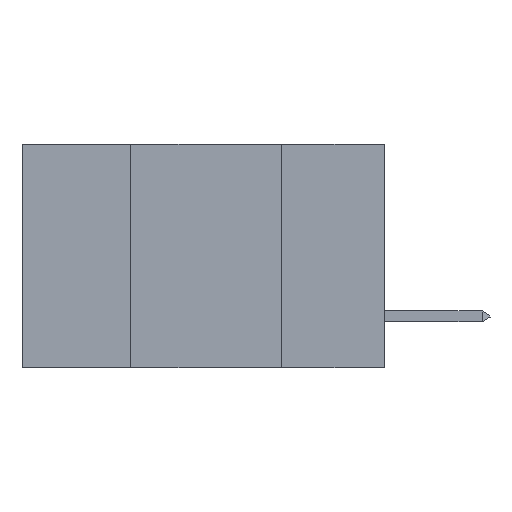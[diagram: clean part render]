
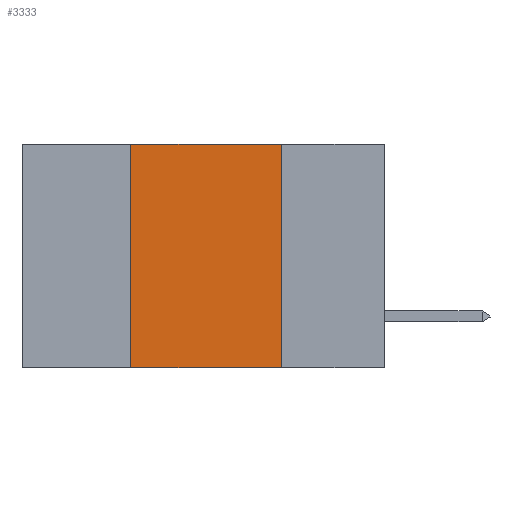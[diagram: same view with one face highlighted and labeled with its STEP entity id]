
A CAD part, left-side view. The second image highlights one B-rep face of the part: STEP entity #3333.
In plain terms, the highlighted planar face has unit normal (-1, 0, 0).
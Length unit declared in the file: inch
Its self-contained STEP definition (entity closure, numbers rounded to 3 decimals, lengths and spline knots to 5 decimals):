
#1678 = VERTEX_POINT ( 'NONE', #30557 ) ;
#2761 = DIRECTION ( 'NONE',  ( 0., -1., 0. ) ) ;
#3333 = ADVANCED_FACE ( 'NONE', ( #39121 ), #10931, .F. ) ;
#3868 = DIRECTION ( 'NONE',  ( 0., 0., -1. ) ) ;
#5580 = VECTOR ( 'NONE', #2761, 39.37008 ) ;
#7299 = CARTESIAN_POINT ( 'NONE',  ( 0., 0.17, 0. ) ) ;
#10762 = CARTESIAN_POINT ( 'NONE',  ( 0., 0.6, -0.37 ) ) ;
#10931 = PLANE ( 'NONE',  #16946 ) ;
#11097 = EDGE_CURVE ( 'NONE', #12855, #47499, #28608, .T. ) ;
#12492 = ORIENTED_EDGE ( 'NONE', *, *, #15811, .F. ) ;
#12855 = VERTEX_POINT ( 'NONE', #33168 ) ;
#14187 = DIRECTION ( 'NONE',  ( 0., -1., 0. ) ) ;
#14217 = CARTESIAN_POINT ( 'NONE',  ( 0., 0.42, 0. ) ) ;
#14856 = DIRECTION ( 'NONE',  ( 0., 0., -1. ) ) ;
#15482 = LINE ( 'NONE', #7299, #34998 ) ;
#15811 = EDGE_CURVE ( 'NONE', #47499, #33558, #34415, .T. ) ;
#16487 = DIRECTION ( 'NONE',  ( 0., 0., 1. ) ) ;
#16946 = AXIS2_PLACEMENT_3D ( 'NONE', #41458, #33560, #14856 ) ;
#19000 = EDGE_CURVE ( 'NONE', #33558, #1678, #15482, .T. ) ;
#20549 = CARTESIAN_POINT ( 'NONE',  ( 0., 0.6, 0. ) ) ;
#22867 = VECTOR ( 'NONE', #14187, 39.37008 ) ;
#23274 = LINE ( 'NONE', #10762, #5580 ) ;
#28608 = LINE ( 'NONE', #40212, #29803 ) ;
#29503 = CARTESIAN_POINT ( 'NONE',  ( 0., 0.17, 0. ) ) ;
#29803 = VECTOR ( 'NONE', #16487, 39.37008 ) ;
#30557 = CARTESIAN_POINT ( 'NONE',  ( 0., 0.17, -0.37 ) ) ;
#32874 = ORIENTED_EDGE ( 'NONE', *, *, #39877, .T. ) ;
#33168 = CARTESIAN_POINT ( 'NONE',  ( 0., 0.42, -0.37 ) ) ;
#33558 = VERTEX_POINT ( 'NONE', #29503 ) ;
#33560 = DIRECTION ( 'NONE',  ( 1., 0., 0. ) ) ;
#34415 = LINE ( 'NONE', #20549, #22867 ) ;
#34998 = VECTOR ( 'NONE', #3868, 39.37008 ) ;
#39121 = FACE_OUTER_BOUND ( 'NONE', #47357, .T. ) ;
#39877 = EDGE_CURVE ( 'NONE', #12855, #1678, #23274, .T. ) ;
#40212 = CARTESIAN_POINT ( 'NONE',  ( 0., 0.42, 0. ) ) ;
#41458 = CARTESIAN_POINT ( 'NONE',  ( 0., 0.6, 0. ) ) ;
#47357 = EDGE_LOOP ( 'NONE', ( #47961, #12492, #49104, #32874 ) ) ;
#47499 = VERTEX_POINT ( 'NONE', #14217 ) ;
#47961 = ORIENTED_EDGE ( 'NONE', *, *, #19000, .F. ) ;
#49104 = ORIENTED_EDGE ( 'NONE', *, *, #11097, .F. ) ;
